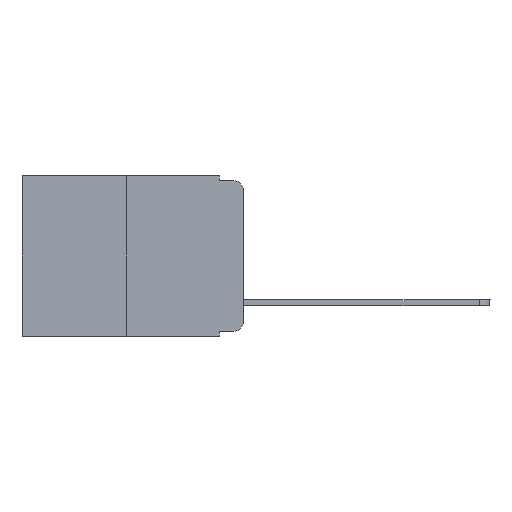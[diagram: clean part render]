
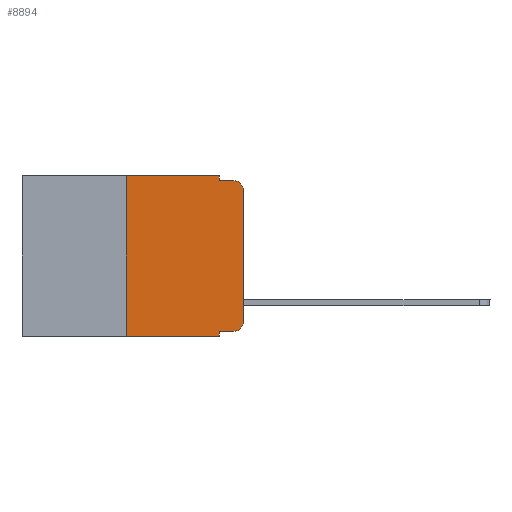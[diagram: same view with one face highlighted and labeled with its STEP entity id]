
A CAD part, left-side view. The second image highlights one B-rep face of the part: STEP entity #8894.
In plain terms, the highlighted planar face has unit normal (-1, 0, 0).
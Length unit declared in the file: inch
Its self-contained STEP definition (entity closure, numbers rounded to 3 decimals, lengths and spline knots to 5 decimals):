
#503 = ORIENTED_EDGE ( 'NONE', *, *, #13623, .F. ) ;
#505 = CARTESIAN_POINT ( 'NONE',  ( 0., 0.473, -0.343 ) ) ;
#519 = VERTEX_POINT ( 'NONE', #6511 ) ;
#538 = DIRECTION ( 'NONE',  ( 0., 0., 1. ) ) ;
#1250 = CARTESIAN_POINT ( 'NONE',  ( 0., 0.051, -0.01 ) ) ;
#1301 = AXIS2_PLACEMENT_3D ( 'NONE', #8232, #14999, #3888 ) ;
#1376 = VERTEX_POINT ( 'NONE', #15215 ) ;
#1581 = CIRCLE ( 'NONE', #11562, 0.02 ) ;
#1591 = EDGE_CURVE ( 'NONE', #5182, #7801, #10944, .T. ) ;
#1912 = EDGE_CURVE ( 'NONE', #6187, #8261, #1581, .T. ) ;
#2206 = EDGE_LOOP ( 'NONE', ( #17356, #17545, #10329, #4746, #503, #17532, #4505, #12596, #8936, #17783 ) ) ;
#2354 = VERTEX_POINT ( 'NONE', #7734 ) ;
#2435 = VERTEX_POINT ( 'NONE', #5132 ) ;
#2545 = LINE ( 'NONE', #505, #4947 ) ;
#2747 = DIRECTION ( 'NONE',  ( 1., 0., 0. ) ) ;
#3062 = VECTOR ( 'NONE', #7314, 39.37008 ) ;
#3244 = EDGE_CURVE ( 'NONE', #5016, #1376, #8305, .T. ) ;
#3888 = DIRECTION ( 'NONE',  ( 0., 0., -1. ) ) ;
#4074 = EDGE_CURVE ( 'NONE', #15994, #6187, #15484, .T. ) ;
#4207 = AXIS2_PLACEMENT_3D ( 'NONE', #15102, #2747, #6786 ) ;
#4505 = ORIENTED_EDGE ( 'NONE', *, *, #14686, .T. ) ;
#4668 = DIRECTION ( 'NONE',  ( 0., 0., -1. ) ) ;
#4706 = CARTESIAN_POINT ( 'NONE',  ( 0., 0., -0.03 ) ) ;
#4746 = ORIENTED_EDGE ( 'NONE', *, *, #12380, .F. ) ;
#4947 = VECTOR ( 'NONE', #10001, 39.37008 ) ;
#5016 = VERTEX_POINT ( 'NONE', #5957 ) ;
#5132 = CARTESIAN_POINT ( 'NONE',  ( 0., 0.051, -0.01 ) ) ;
#5182 = VERTEX_POINT ( 'NONE', #6086 ) ;
#5957 = CARTESIAN_POINT ( 'NONE',  ( 0., 0.25, -0.343 ) ) ;
#6086 = CARTESIAN_POINT ( 'NONE',  ( 0., 0.051, -0.333 ) ) ;
#6187 = VERTEX_POINT ( 'NONE', #4706 ) ;
#6433 = CARTESIAN_POINT ( 'NONE',  ( 0., 0.051, 0. ) ) ;
#6511 = CARTESIAN_POINT ( 'NONE',  ( 0., 0.051, -0.343 ) ) ;
#6708 = CARTESIAN_POINT ( 'NONE',  ( 0., 0.051, -0.333 ) ) ;
#6786 = DIRECTION ( 'NONE',  ( 0., 0., -1. ) ) ;
#7314 = DIRECTION ( 'NONE',  ( 0., 0., -1. ) ) ;
#7320 = CARTESIAN_POINT ( 'NONE',  ( 0., 0.02, -0.01 ) ) ;
#7734 = CARTESIAN_POINT ( 'NONE',  ( 0., 0.051, 0. ) ) ;
#7801 = VERTEX_POINT ( 'NONE', #16920 ) ;
#8014 = DIRECTION ( 'NONE',  ( 0., -1., 0. ) ) ;
#8118 = DIRECTION ( 'NONE',  ( 0., -1., 0. ) ) ;
#8232 = CARTESIAN_POINT ( 'NONE',  ( 0., 0.02, -0.313 ) ) ;
#8261 = VERTEX_POINT ( 'NONE', #7320 ) ;
#8270 = PLANE ( 'NONE',  #4207 ) ;
#8305 = LINE ( 'NONE', #11255, #12661 ) ;
#8894 = ADVANCED_FACE ( 'NONE', ( #9114 ), #8270, .F. ) ;
#8936 = ORIENTED_EDGE ( 'NONE', *, *, #1591, .T. ) ;
#9114 = FACE_OUTER_BOUND ( 'NONE', #2206, .T. ) ;
#9938 = CIRCLE ( 'NONE', #1301, 0.02 ) ;
#9968 = CARTESIAN_POINT ( 'NONE',  ( 0., 0.473, 0. ) ) ;
#10001 = DIRECTION ( 'NONE',  ( 0., -1., 0. ) ) ;
#10261 = EDGE_CURVE ( 'NONE', #2435, #8261, #16305, .T. ) ;
#10275 = EDGE_CURVE ( 'NONE', #7801, #15994, #9938, .T. ) ;
#10296 = CARTESIAN_POINT ( 'NONE',  ( 0., 0.02, -0.03 ) ) ;
#10329 = ORIENTED_EDGE ( 'NONE', *, *, #10261, .F. ) ;
#10450 = LINE ( 'NONE', #15479, #3062 ) ;
#10679 = VECTOR ( 'NONE', #538, 39.37008 ) ;
#10944 = LINE ( 'NONE', #6708, #17535 ) ;
#11255 = CARTESIAN_POINT ( 'NONE',  ( 0., 0.25, 0. ) ) ;
#11554 = CARTESIAN_POINT ( 'NONE',  ( 0., 0., -0.313 ) ) ;
#11562 = AXIS2_PLACEMENT_3D ( 'NONE', #10296, #13123, #4668 ) ;
#12155 = VECTOR ( 'NONE', #13991, 39.37008 ) ;
#12380 = EDGE_CURVE ( 'NONE', #2354, #2435, #10450, .T. ) ;
#12546 = VECTOR ( 'NONE', #8118, 39.37008 ) ;
#12550 = VECTOR ( 'NONE', #13336, 39.37008 ) ;
#12596 = ORIENTED_EDGE ( 'NONE', *, *, #13912, .F. ) ;
#12661 = VECTOR ( 'NONE', #15373, 39.37008 ) ;
#13123 = DIRECTION ( 'NONE',  ( -1., 0., 0. ) ) ;
#13336 = DIRECTION ( 'NONE',  ( 0., 0., -1. ) ) ;
#13623 = EDGE_CURVE ( 'NONE', #1376, #2354, #14981, .T. ) ;
#13674 = LINE ( 'NONE', #6433, #12550 ) ;
#13912 = EDGE_CURVE ( 'NONE', #5182, #519, #13674, .T. ) ;
#13991 = DIRECTION ( 'NONE',  ( 0., -1., 0. ) ) ;
#14686 = EDGE_CURVE ( 'NONE', #5016, #519, #2545, .T. ) ;
#14981 = LINE ( 'NONE', #9968, #12155 ) ;
#14999 = DIRECTION ( 'NONE',  ( -1., 0., 0. ) ) ;
#15102 = CARTESIAN_POINT ( 'NONE',  ( 0., 0.473, 0. ) ) ;
#15215 = CARTESIAN_POINT ( 'NONE',  ( 0., 0.25, 0. ) ) ;
#15373 = DIRECTION ( 'NONE',  ( 0., 0., 1. ) ) ;
#15479 = CARTESIAN_POINT ( 'NONE',  ( 0., 0.051, 0. ) ) ;
#15484 = LINE ( 'NONE', #17246, #10679 ) ;
#15994 = VERTEX_POINT ( 'NONE', #11554 ) ;
#16305 = LINE ( 'NONE', #1250, #12546 ) ;
#16920 = CARTESIAN_POINT ( 'NONE',  ( 0., 0.02, -0.333 ) ) ;
#17246 = CARTESIAN_POINT ( 'NONE',  ( 0., 0., 0. ) ) ;
#17356 = ORIENTED_EDGE ( 'NONE', *, *, #4074, .T. ) ;
#17532 = ORIENTED_EDGE ( 'NONE', *, *, #3244, .F. ) ;
#17535 = VECTOR ( 'NONE', #8014, 39.37008 ) ;
#17545 = ORIENTED_EDGE ( 'NONE', *, *, #1912, .T. ) ;
#17783 = ORIENTED_EDGE ( 'NONE', *, *, #10275, .T. ) ;
